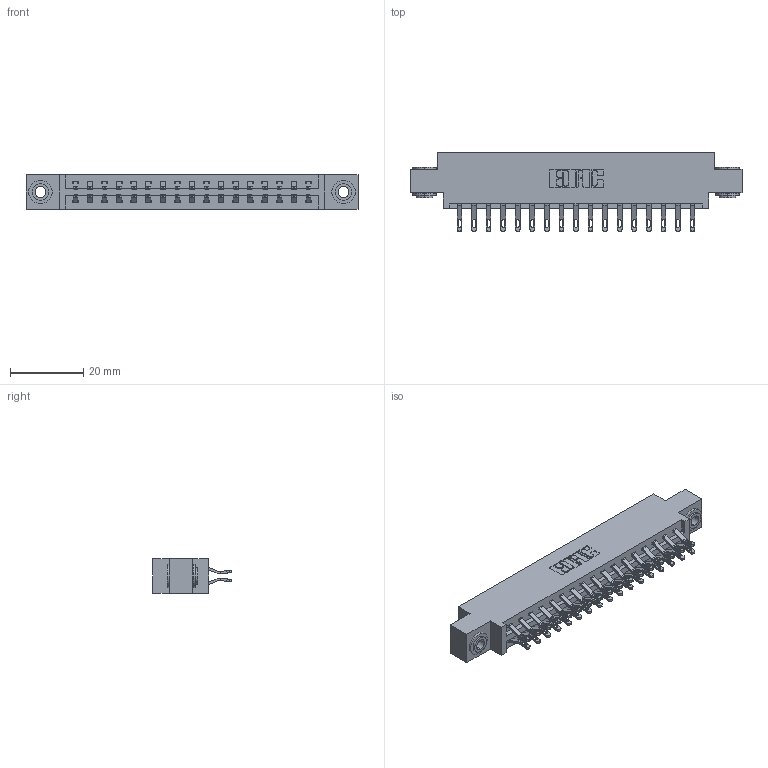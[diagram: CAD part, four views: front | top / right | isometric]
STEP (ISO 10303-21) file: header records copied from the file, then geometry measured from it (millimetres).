
FILE_DESCRIPTION (( 'STEP AP203' ), '1' );
FILE_NAME ('337-034-555-803.STEP', '2018-08-07T13:11:07', ( '' ), ( '' ), 'SwSTEP 2.0', 'SolidWorks 2016', '' );
FILE_SCHEMA (( 'CONFIG_CONTROL_DESIGN' ));
Length unit declared in the file: inch
Products named in the file (4): 337-034-555-803; 337 Part_0.170 Offset - 0.156 Dia-TH; 345-292-001_555 Tail; 345-250-002_345-250-002-102
Assembly tree (37 placements, depth 2):
  337-034-555-803
    337 Part_0.170 Offset - 0.156 Dia-TH
    345-292-001_555 Tail  x34
    345-250-002_345-250-002-102  x2
Bounding box: 90.37 x 21.47 x 9.4 mm (x, y, z)
Volume: 9192 mm3; surface area: 10852.6 mm2
Topology: 37 solids, 37 shells, 2196 faces, 6825 edges, 4546 vertices
Faces by surface type: plane 1308, cylinder 880, cone 8
Entity records: 17522 total; most frequent: CARTESIAN_POINT 2983, ORIENTED_EDGE 2882, DIRECTION 2587, EDGE_CURVE 1441, VECTOR 1269, LINE 1269, VERTEX_POINT 958, AXIS2_PLACEMENT_3D 659
